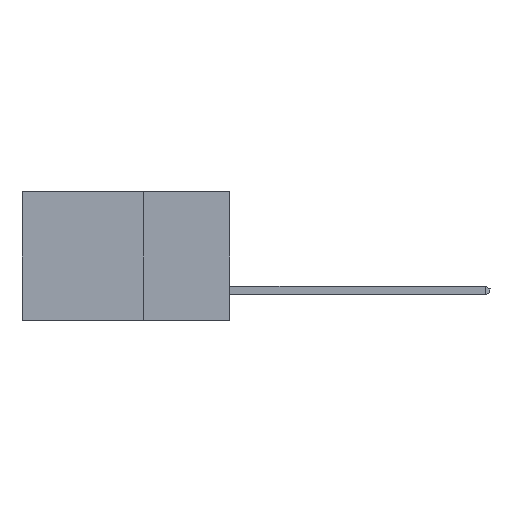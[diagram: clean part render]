
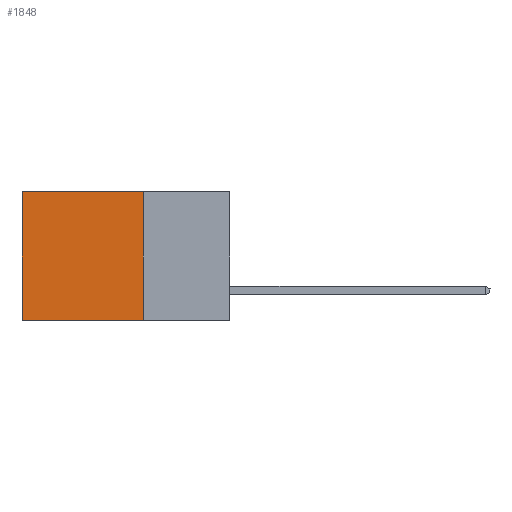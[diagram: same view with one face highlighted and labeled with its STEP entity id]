
A CAD part, left-side view. The second image highlights one B-rep face of the part: STEP entity #1848.
In plain terms, the highlighted planar face has unit normal (-1, 0, 0).
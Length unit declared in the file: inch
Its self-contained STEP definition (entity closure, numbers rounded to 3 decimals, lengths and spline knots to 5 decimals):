
#213 = CARTESIAN_POINT ( 'NONE',  ( 0.2615, 0.25, -0.37 ) ) ;
#493 = DIRECTION ( 'NONE',  ( 0., 1., 0. ) ) ;
#613 = EDGE_CURVE ( 'NONE', #1374, #6371, #2250, .T. ) ;
#679 = EDGE_CURVE ( 'NONE', #8920, #9107, #4333, .T. ) ;
#939 = CARTESIAN_POINT ( 'NONE',  ( 0.2615, 0.6, -0.37 ) ) ;
#1090 = DIRECTION ( 'NONE',  ( 0., 0., -1. ) ) ;
#1136 = EDGE_LOOP ( 'NONE', ( #2800, #4372, #4572, #10047 ) ) ;
#1357 = VECTOR ( 'NONE', #493, 39.37008 ) ;
#1374 = VERTEX_POINT ( 'NONE', #6038 ) ;
#1848 = ADVANCED_FACE ( 'NONE', ( #9516 ), #2368, .F. ) ;
#1955 = VECTOR ( 'NONE', #11436, 39.37008 ) ;
#1958 = LINE ( 'NONE', #5230, #5078 ) ;
#2250 = LINE ( 'NONE', #4924, #1357 ) ;
#2368 = PLANE ( 'NONE',  #6565 ) ;
#2800 = ORIENTED_EDGE ( 'NONE', *, *, #3626, .T. ) ;
#3626 = EDGE_CURVE ( 'NONE', #6371, #9107, #9798, .T. ) ;
#4085 = CARTESIAN_POINT ( 'NONE',  ( 0.2615, 0.6, 0. ) ) ;
#4333 = LINE ( 'NONE', #213, #1955 ) ;
#4372 = ORIENTED_EDGE ( 'NONE', *, *, #679, .F. ) ;
#4572 = ORIENTED_EDGE ( 'NONE', *, *, #6407, .F. ) ;
#4657 = CARTESIAN_POINT ( 'NONE',  ( 0.2615, 0.6, -0.37 ) ) ;
#4924 = CARTESIAN_POINT ( 'NONE',  ( 0.2615, 0.25, 0. ) ) ;
#5036 = DIRECTION ( 'NONE',  ( 0., 0., -1. ) ) ;
#5078 = VECTOR ( 'NONE', #1090, 39.37008 ) ;
#5230 = CARTESIAN_POINT ( 'NONE',  ( 0.2615, 0.25, -0.37 ) ) ;
#5414 = DIRECTION ( 'NONE',  ( 0., 0., -1. ) ) ;
#5907 = CARTESIAN_POINT ( 'NONE',  ( 0.2615, 0.25, -0.37 ) ) ;
#5959 = DIRECTION ( 'NONE',  ( 1., 0., 0. ) ) ;
#6038 = CARTESIAN_POINT ( 'NONE',  ( 0.2615, 0.25, 0. ) ) ;
#6371 = VERTEX_POINT ( 'NONE', #4085 ) ;
#6407 = EDGE_CURVE ( 'NONE', #1374, #8920, #1958, .T. ) ;
#6565 = AXIS2_PLACEMENT_3D ( 'NONE', #5907, #5959, #5036 ) ;
#6596 = VECTOR ( 'NONE', #5414, 39.37008 ) ;
#7987 = CARTESIAN_POINT ( 'NONE',  ( 0.2615, 0.25, -0.37 ) ) ;
#8920 = VERTEX_POINT ( 'NONE', #7987 ) ;
#9107 = VERTEX_POINT ( 'NONE', #4657 ) ;
#9516 = FACE_OUTER_BOUND ( 'NONE', #1136, .T. ) ;
#9798 = LINE ( 'NONE', #939, #6596 ) ;
#10047 = ORIENTED_EDGE ( 'NONE', *, *, #613, .T. ) ;
#11436 = DIRECTION ( 'NONE',  ( 0., 1., 0. ) ) ;
